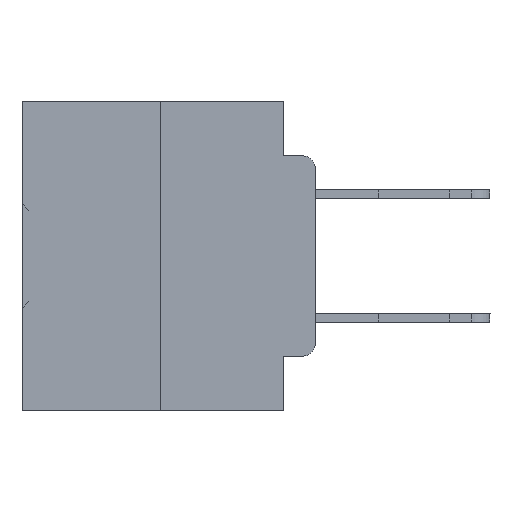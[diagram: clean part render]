
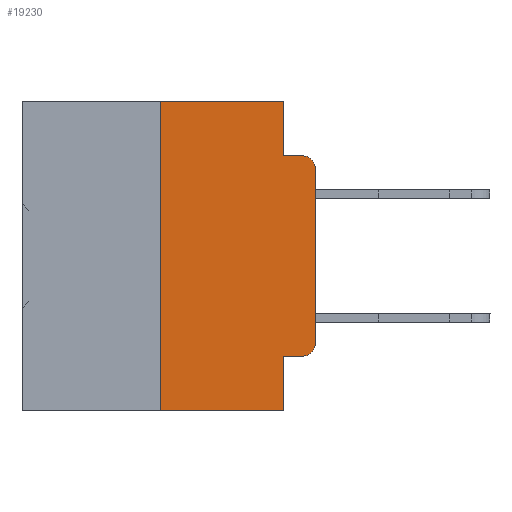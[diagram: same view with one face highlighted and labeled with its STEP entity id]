
A CAD part, left-side view. The second image highlights one B-rep face of the part: STEP entity #19230.
In plain terms, the highlighted planar face has unit normal (-1, 0, 0).
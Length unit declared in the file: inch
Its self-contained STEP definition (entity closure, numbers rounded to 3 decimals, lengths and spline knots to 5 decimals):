
#486 = ORIENTED_EDGE ( 'NONE', *, *, #14578, .F. ) ;
#794 = ORIENTED_EDGE ( 'NONE', *, *, #18122, .F. ) ;
#1158 = ORIENTED_EDGE ( 'NONE', *, *, #9539, .T. ) ;
#1652 = DIRECTION ( 'NONE',  ( 0., 0., 1. ) ) ;
#2667 = CARTESIAN_POINT ( 'NONE',  ( 0., 0.051, -0.4115 ) ) ;
#3558 = CARTESIAN_POINT ( 'NONE',  ( 0., 0.051, 0. ) ) ;
#3768 = CARTESIAN_POINT ( 'NONE',  ( 0., 0.02, -0.1085 ) ) ;
#5165 = CARTESIAN_POINT ( 'NONE',  ( 0., 0., -0.3915 ) ) ;
#5469 = CARTESIAN_POINT ( 'NONE',  ( 0., 0.25, -0.5 ) ) ;
#5797 = DIRECTION ( 'NONE',  ( 1., 0., 0. ) ) ;
#6408 = LINE ( 'NONE', #23300, #14396 ) ;
#7288 = FACE_OUTER_BOUND ( 'NONE', #21349, .T. ) ;
#7762 = CARTESIAN_POINT ( 'NONE',  ( 0., 0., 0. ) ) ;
#7845 = VERTEX_POINT ( 'NONE', #3558 ) ;
#8170 = CARTESIAN_POINT ( 'NONE',  ( 0., 0.051, -0.5 ) ) ;
#8382 = AXIS2_PLACEMENT_3D ( 'NONE', #3768, #31750, #37814 ) ;
#8653 = DIRECTION ( 'NONE',  ( 0., 0., -1. ) ) ;
#8720 = DIRECTION ( 'NONE',  ( 0., -1., 0. ) ) ;
#9539 = EDGE_CURVE ( 'NONE', #24234, #19759, #12664, .T. ) ;
#9699 = ORIENTED_EDGE ( 'NONE', *, *, #26913, .T. ) ;
#10144 = VERTEX_POINT ( 'NONE', #32424 ) ;
#11494 = DIRECTION ( 'NONE',  ( -1., 0., 0. ) ) ;
#11796 = VECTOR ( 'NONE', #8720, 39.37008 ) ;
#11832 = LINE ( 'NONE', #26318, #12703 ) ;
#12664 = LINE ( 'NONE', #2667, #11796 ) ;
#12703 = VECTOR ( 'NONE', #13931, 39.37008 ) ;
#13635 = DIRECTION ( 'NONE',  ( 0., -1., 0. ) ) ;
#13931 = DIRECTION ( 'NONE',  ( 0., -1., 0. ) ) ;
#14396 = VECTOR ( 'NONE', #26322, 39.37008 ) ;
#14578 = EDGE_CURVE ( 'NONE', #23380, #10144, #21260, .T. ) ;
#14643 = VECTOR ( 'NONE', #1652, 39.37008 ) ;
#14766 = CARTESIAN_POINT ( 'NONE',  ( 0., 0.02, -0.3915 ) ) ;
#15035 = AXIS2_PLACEMENT_3D ( 'NONE', #14766, #11494, #8653 ) ;
#15559 = EDGE_CURVE ( 'NONE', #10144, #7845, #11832, .T. ) ;
#15637 = AXIS2_PLACEMENT_3D ( 'NONE', #20752, #5797, #26779 ) ;
#15707 = CARTESIAN_POINT ( 'NONE',  ( 0., 0.051, -0.4115 ) ) ;
#15808 = VECTOR ( 'NONE', #18952, 39.37008 ) ;
#15957 = ORIENTED_EDGE ( 'NONE', *, *, #28896, .T. ) ;
#16426 = CARTESIAN_POINT ( 'NONE',  ( 0., 0.25, 0. ) ) ;
#18122 = EDGE_CURVE ( 'NONE', #27024, #37675, #6408, .T. ) ;
#18695 = CARTESIAN_POINT ( 'NONE',  ( 0., 0.02, -0.4115 ) ) ;
#18952 = DIRECTION ( 'NONE',  ( 0., 0., -1. ) ) ;
#19230 = ADVANCED_FACE ( 'NONE', ( #7288 ), #35463, .F. ) ;
#19759 = VERTEX_POINT ( 'NONE', #18695 ) ;
#20522 = ORIENTED_EDGE ( 'NONE', *, *, #33779, .F. ) ;
#20752 = CARTESIAN_POINT ( 'NONE',  ( 0., 0.473, 0. ) ) ;
#21100 = VERTEX_POINT ( 'NONE', #21770 ) ;
#21260 = LINE ( 'NONE', #16426, #14643 ) ;
#21349 = EDGE_LOOP ( 'NONE', ( #9699, #21631, #794, #20522, #27541, #486, #15957, #23729, #1158, #32886 ) ) ;
#21631 = ORIENTED_EDGE ( 'NONE', *, *, #27966, .T. ) ;
#21643 = VECTOR ( 'NONE', #13635, 39.37008 ) ;
#21767 = EDGE_CURVE ( 'NONE', #24234, #22795, #23479, .T. ) ;
#21770 = CARTESIAN_POINT ( 'NONE',  ( 0., 0., -0.1085 ) ) ;
#22506 = VECTOR ( 'NONE', #34364, 39.37008 ) ;
#22795 = VERTEX_POINT ( 'NONE', #8170 ) ;
#22813 = CARTESIAN_POINT ( 'NONE',  ( 0., 0.051, -0.0885 ) ) ;
#23300 = CARTESIAN_POINT ( 'NONE',  ( 0., 0.051, -0.0885 ) ) ;
#23380 = VERTEX_POINT ( 'NONE', #5469 ) ;
#23479 = LINE ( 'NONE', #37797, #22506 ) ;
#23729 = ORIENTED_EDGE ( 'NONE', *, *, #21767, .F. ) ;
#24234 = VERTEX_POINT ( 'NONE', #15707 ) ;
#24483 = CIRCLE ( 'NONE', #8382, 0.02 ) ;
#24731 = EDGE_CURVE ( 'NONE', #19759, #26931, #35919, .T. ) ;
#25592 = DIRECTION ( 'NONE',  ( 0., 0., 1. ) ) ;
#26318 = CARTESIAN_POINT ( 'NONE',  ( 0., 0.473, 0. ) ) ;
#26322 = DIRECTION ( 'NONE',  ( 0., -1., 0. ) ) ;
#26779 = DIRECTION ( 'NONE',  ( 0., 0., -1. ) ) ;
#26913 = EDGE_CURVE ( 'NONE', #26931, #21100, #38269, .T. ) ;
#26931 = VERTEX_POINT ( 'NONE', #5165 ) ;
#27024 = VERTEX_POINT ( 'NONE', #22813 ) ;
#27541 = ORIENTED_EDGE ( 'NONE', *, *, #15559, .F. ) ;
#27966 = EDGE_CURVE ( 'NONE', #21100, #37675, #24483, .T. ) ;
#28842 = CARTESIAN_POINT ( 'NONE',  ( 0., 0.473, -0.5 ) ) ;
#28896 = EDGE_CURVE ( 'NONE', #23380, #22795, #29692, .T. ) ;
#29358 = VECTOR ( 'NONE', #25592, 39.37008 ) ;
#29692 = LINE ( 'NONE', #28842, #21643 ) ;
#31750 = DIRECTION ( 'NONE',  ( -1., 0., 0. ) ) ;
#31862 = LINE ( 'NONE', #37107, #15808 ) ;
#32424 = CARTESIAN_POINT ( 'NONE',  ( 0., 0.25, 0. ) ) ;
#32886 = ORIENTED_EDGE ( 'NONE', *, *, #24731, .T. ) ;
#33779 = EDGE_CURVE ( 'NONE', #7845, #27024, #31862, .T. ) ;
#33950 = CARTESIAN_POINT ( 'NONE',  ( 0., 0.02, -0.0885 ) ) ;
#34364 = DIRECTION ( 'NONE',  ( 0., 0., -1. ) ) ;
#35463 = PLANE ( 'NONE',  #15637 ) ;
#35919 = CIRCLE ( 'NONE', #15035, 0.02 ) ;
#37107 = CARTESIAN_POINT ( 'NONE',  ( 0., 0.051, 0. ) ) ;
#37675 = VERTEX_POINT ( 'NONE', #33950 ) ;
#37797 = CARTESIAN_POINT ( 'NONE',  ( 0., 0.051, 0. ) ) ;
#37814 = DIRECTION ( 'NONE',  ( 0., 0., -1. ) ) ;
#38269 = LINE ( 'NONE', #7762, #29358 ) ;
